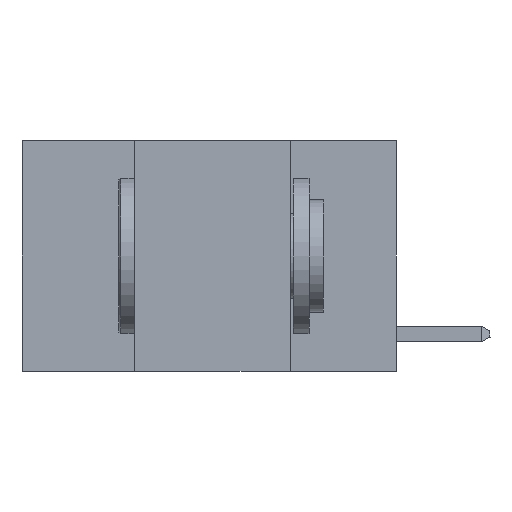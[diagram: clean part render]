
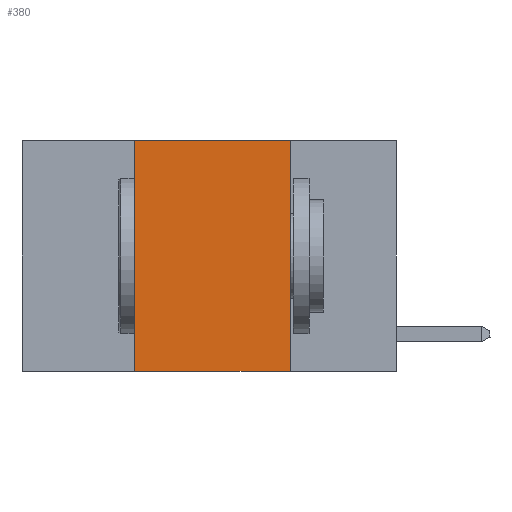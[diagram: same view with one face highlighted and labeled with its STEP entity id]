
A CAD part, left-side view. The second image highlights one B-rep face of the part: STEP entity #380.
In plain terms, the highlighted planar face has unit normal (-1, 0, 0).
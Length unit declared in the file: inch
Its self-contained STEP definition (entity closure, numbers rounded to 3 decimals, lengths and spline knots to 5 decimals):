
#380 = ADVANCED_FACE ( 'NONE', ( #11469 ), #1490, .F. ) ;
#694 = DIRECTION ( 'NONE',  ( 0., 0., 1. ) ) ;
#840 = CARTESIAN_POINT ( 'NONE',  ( 0., 0.17, 0. ) ) ;
#904 = DIRECTION ( 'NONE',  ( 0., 0., -1. ) ) ;
#1050 = DIRECTION ( 'NONE',  ( 1., 0., 0. ) ) ;
#1217 = VERTEX_POINT ( 'NONE', #840 ) ;
#1318 = EDGE_CURVE ( 'NONE', #4451, #1217, #5367, .T. ) ;
#1490 = PLANE ( 'NONE',  #3213 ) ;
#1707 = ORIENTED_EDGE ( 'NONE', *, *, #15661, .F. ) ;
#1840 = DIRECTION ( 'NONE',  ( 0., -1., 0. ) ) ;
#1869 = LINE ( 'NONE', #15209, #11197 ) ;
#2205 = EDGE_CURVE ( 'NONE', #10440, #2714, #8569, .T. ) ;
#2324 = CARTESIAN_POINT ( 'NONE',  ( 0., 0.6, 0. ) ) ;
#2714 = VERTEX_POINT ( 'NONE', #6579 ) ;
#2967 = CARTESIAN_POINT ( 'NONE',  ( 0., 0.42, -0.37 ) ) ;
#3213 = AXIS2_PLACEMENT_3D ( 'NONE', #2324, #1050, #904 ) ;
#3418 = LINE ( 'NONE', #10269, #15467 ) ;
#4451 = VERTEX_POINT ( 'NONE', #6267 ) ;
#4937 = ORIENTED_EDGE ( 'NONE', *, *, #1318, .F. ) ;
#5367 = LINE ( 'NONE', #10326, #14242 ) ;
#6267 = CARTESIAN_POINT ( 'NONE',  ( 0., 0.42, 0. ) ) ;
#6579 = CARTESIAN_POINT ( 'NONE',  ( 0., 0.17, -0.37 ) ) ;
#8513 = ORIENTED_EDGE ( 'NONE', *, *, #2205, .T. ) ;
#8569 = LINE ( 'NONE', #9098, #11058 ) ;
#9098 = CARTESIAN_POINT ( 'NONE',  ( 0., 0.6, -0.37 ) ) ;
#9772 = DIRECTION ( 'NONE',  ( 0., -1., 0. ) ) ;
#10269 = CARTESIAN_POINT ( 'NONE',  ( 0., 0.17, 0. ) ) ;
#10326 = CARTESIAN_POINT ( 'NONE',  ( 0., 0.6, 0. ) ) ;
#10440 = VERTEX_POINT ( 'NONE', #2967 ) ;
#11058 = VECTOR ( 'NONE', #1840, 39.37008 ) ;
#11197 = VECTOR ( 'NONE', #694, 39.37008 ) ;
#11245 = EDGE_CURVE ( 'NONE', #10440, #4451, #1869, .T. ) ;
#11469 = FACE_OUTER_BOUND ( 'NONE', #11493, .T. ) ;
#11493 = EDGE_LOOP ( 'NONE', ( #1707, #4937, #14131, #8513 ) ) ;
#11500 = DIRECTION ( 'NONE',  ( 0., 0., -1. ) ) ;
#14131 = ORIENTED_EDGE ( 'NONE', *, *, #11245, .F. ) ;
#14242 = VECTOR ( 'NONE', #9772, 39.37008 ) ;
#15209 = CARTESIAN_POINT ( 'NONE',  ( 0., 0.42, 0. ) ) ;
#15467 = VECTOR ( 'NONE', #11500, 39.37008 ) ;
#15661 = EDGE_CURVE ( 'NONE', #1217, #2714, #3418, .T. ) ;
